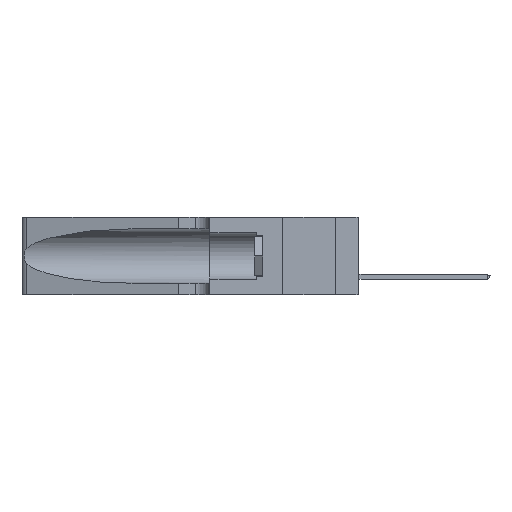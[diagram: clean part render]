
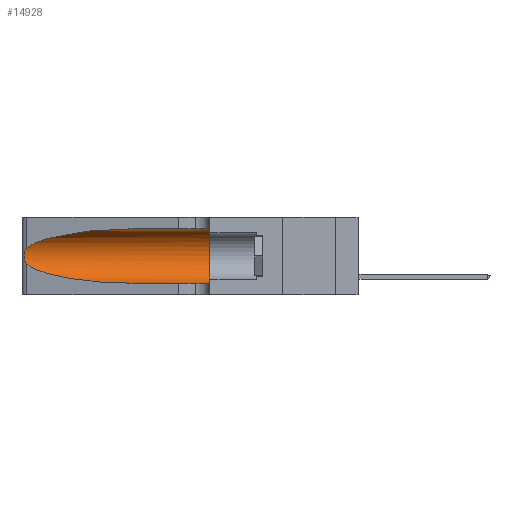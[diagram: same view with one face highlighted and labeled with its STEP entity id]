
A CAD part, left-side view. The second image highlights one B-rep face of the part: STEP entity #14928.
In plain terms, the highlighted cylindrical face has radius 3.308 mm (diameter 6.617 mm), a partial arc.
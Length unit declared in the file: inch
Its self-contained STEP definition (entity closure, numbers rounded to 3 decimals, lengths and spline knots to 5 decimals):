
#930 = LINE ( 'NONE', #39347, #35647 ) ;
#1129 = CARTESIAN_POINT ( 'NONE',  ( 0.26075, 1.23896, 0.178 ) ) ;
#1397 = AXIS2_PLACEMENT_3D ( 'NONE', #41966, #24177, #45796 ) ;
#2801 = ORIENTED_EDGE ( 'NONE', *, *, #34968, .T. ) ;
#4593 = CYLINDRICAL_SURFACE ( 'NONE', #1397, 0.13025 ) ;
#5681 = ORIENTED_EDGE ( 'NONE', *, *, #43511, .T. ) ;
#5944 = CARTESIAN_POINT ( 'NONE',  ( 0.1305, 0.72297, 0.05475 ) ) ;
#5994 = CARTESIAN_POINT ( 'NONE',  ( 0.1305, 0.35, 0.05475 ) ) ;
#7939 = DIRECTION ( 'NONE',  ( 0., 0., 1. ) ) ;
#8112 = VERTEX_POINT ( 'NONE', #17293 ) ;
#8433 = CARTESIAN_POINT ( 'NONE',  ( 0.18966, 0.96281, 0.05475 ) ) ;
#9207 = CARTESIAN_POINT ( 'NONE',  ( 0.1305, 0.72297, 0.31525 ) ) ;
#11776 = VERTEX_POINT ( 'NONE', #37174 ) ;
#11957 = CARTESIAN_POINT ( 'NONE',  ( 0.26018, 1.23835, 0.19895 ) ) ;
#12188 = ORIENTED_EDGE ( 'NONE', *, *, #22642, .T. ) ;
#13332 = CIRCLE ( 'NONE', #20176, 0.13025 ) ;
#14928 = ADVANCED_FACE ( 'NONE', ( #25006 ), #4593, .F. ) ;
#15931 = CARTESIAN_POINT ( 'NONE',  ( 0.26017, 1.23833, 0.17102 ) ) ;
#16357 = CARTESIAN_POINT ( 'NONE',  ( 0.18966, 0.96281, 0.31525 ) ) ;
#16625 = ORIENTED_EDGE ( 'NONE', *, *, #41782, .F. ) ;
#17293 = CARTESIAN_POINT ( 'NONE',  ( 0.1305, 0.35, 0.31525 ) ) ;
#19043 = CARTESIAN_POINT ( 'NONE',  ( 0.25787, 1.23484, 0.2124 ) ) ;
#19351 = CARTESIAN_POINT ( 'NONE',  ( 0.25639, 1.23186, 0.15144 ) ) ;
#20176 = AXIS2_PLACEMENT_3D ( 'NONE', #30270, #25946, #7939 ) ;
#21683 = EDGE_LOOP ( 'NONE', ( #12188, #5681, #2801, #24202, #46060, #16625 ) ) ;
#22642 = EDGE_CURVE ( 'NONE', #42034, #26850, #33178, .T. ) ;
#22924 = CARTESIAN_POINT ( 'NONE',  ( 0.25487, 1.22718, 0.14631 ) ) ;
#22956 = CARTESIAN_POINT ( 'NONE',  ( 0.25487, 1.22718, 0.14631 ) ) ;
#23088 = CARTESIAN_POINT ( 'NONE',  ( 0.2373, 1.15595, 0.08982 ) ) ;
#23122 = CARTESIAN_POINT ( 'NONE',  ( 0.26075, 1.23896, 0.19203 ) ) ;
#24177 = DIRECTION ( 'NONE',  ( 0., -1., 0. ) ) ;
#24202 = ORIENTED_EDGE ( 'NONE', *, *, #46043, .T. ) ;
#24622 = EDGE_CURVE ( 'NONE', #8112, #42250, #13332, .T. ) ;
#25006 = FACE_OUTER_BOUND ( 'NONE', #21683, .T. ) ;
#25887 = DIRECTION ( 'NONE',  ( 0., -1., 0. ) ) ;
#25946 = DIRECTION ( 'NONE',  ( 0., 1., 0. ) ) ;
#26305 = CARTESIAN_POINT ( 'NONE',  ( 0.25854, 1.2359, 0.20912 ) ) ;
#26850 = VERTEX_POINT ( 'NONE', #30103 ) ;
#26918 = CARTESIAN_POINT ( 'NONE',  ( 0.1305, 0.72297, 0.05475 ) ) ;
#26954 = CARTESIAN_POINT ( 'NONE',  ( 0.25555, 1.22993, 0.14849 ) ) ;
#27960 =( BOUNDED_CURVE ( )  B_SPLINE_CURVE ( 3, ( #22924, #23088, #8433, #26918 ),
 .UNSPECIFIED., .F., .F. ) 
 B_SPLINE_CURVE_WITH_KNOTS ( ( 4, 4 ),
 ( 3.44316, 4.71239 ),
 .UNSPECIFIED. ) 
 CURVE ( )  GEOMETRIC_REPRESENTATION_ITEM ( )  RATIONAL_B_SPLINE_CURVE ( ( 1., 0.87, 0.87, 1. ) ) 
 REPRESENTATION_ITEM ( '' )  );
#29252 = VERTEX_POINT ( 'NONE', #5944 ) ;
#29939 = VECTOR ( 'NONE', #25887, 39.37008 ) ;
#29995 = CARTESIAN_POINT ( 'NONE',  ( 0.25789, 1.23486, 0.15765 ) ) ;
#30103 = CARTESIAN_POINT ( 'NONE',  ( 0.25487, 1.22718, 0.22369 ) ) ;
#30270 = CARTESIAN_POINT ( 'NONE',  ( 0.1305, 0.35, 0.185 ) ) ;
#31066 = CARTESIAN_POINT ( 'NONE',  ( 0.25487, 1.22718, 0.22369 ) ) ;
#32146 = B_SPLINE_CURVE_WITH_KNOTS ( 'NONE', 3,
 ( #33327, #40577, #33948, #19043, #26305, #11957, #23122, #1129, #15931, #37297, #29995, #19351, #26954, #22956 ),
 .UNSPECIFIED., .F., .F.,
 ( 4, 2, 2, 2, 2, 2, 4 ),
 ( 0., 0.00027, 0.00053, 0.00107, 0.0016, 0.00187, 0.00214 ),
 .UNSPECIFIED. ) ;
#32284 = LINE ( 'NONE', #43821, #29939 ) ;
#33178 =( BOUNDED_CURVE ( )  B_SPLINE_CURVE ( 3, ( #9207, #16357, #45289, #31066 ),
 .UNSPECIFIED., .F., .F. ) 
 B_SPLINE_CURVE_WITH_KNOTS ( ( 4, 4 ),
 ( 1.5708, 2.84003 ),
 .UNSPECIFIED. ) 
 CURVE ( )  GEOMETRIC_REPRESENTATION_ITEM ( )  RATIONAL_B_SPLINE_CURVE ( ( 1., 0.87, 0.87, 1. ) ) 
 REPRESENTATION_ITEM ( '' )  );
#33327 = CARTESIAN_POINT ( 'NONE',  ( 0.25487, 1.22718, 0.22369 ) ) ;
#33948 = CARTESIAN_POINT ( 'NONE',  ( 0.25639, 1.23184, 0.21858 ) ) ;
#34968 = EDGE_CURVE ( 'NONE', #11776, #29252, #27960, .T. ) ;
#35647 = VECTOR ( 'NONE', #43283, 39.37008 ) ;
#37174 = CARTESIAN_POINT ( 'NONE',  ( 0.25487, 1.22718, 0.14631 ) ) ;
#37297 = CARTESIAN_POINT ( 'NONE',  ( 0.25856, 1.23593, 0.16098 ) ) ;
#39347 = CARTESIAN_POINT ( 'NONE',  ( 0.1305, 1.61858, 0.05475 ) ) ;
#40577 = CARTESIAN_POINT ( 'NONE',  ( 0.25555, 1.22994, 0.2215 ) ) ;
#41782 = EDGE_CURVE ( 'NONE', #42034, #8112, #32284, .T. ) ;
#41966 = CARTESIAN_POINT ( 'NONE',  ( 0.1305, 1.61858, 0.185 ) ) ;
#42034 = VERTEX_POINT ( 'NONE', #46895 ) ;
#42250 = VERTEX_POINT ( 'NONE', #5994 ) ;
#43283 = DIRECTION ( 'NONE',  ( 0., -1., 0. ) ) ;
#43511 = EDGE_CURVE ( 'NONE', #26850, #11776, #32146, .T. ) ;
#43821 = CARTESIAN_POINT ( 'NONE',  ( 0.1305, 1.61858, 0.31525 ) ) ;
#45289 = CARTESIAN_POINT ( 'NONE',  ( 0.2373, 1.15595, 0.28018 ) ) ;
#45796 = DIRECTION ( 'NONE',  ( 0., 0., -1. ) ) ;
#46043 = EDGE_CURVE ( 'NONE', #29252, #42250, #930, .T. ) ;
#46060 = ORIENTED_EDGE ( 'NONE', *, *, #24622, .F. ) ;
#46895 = CARTESIAN_POINT ( 'NONE',  ( 0.1305, 0.72297, 0.31525 ) ) ;
